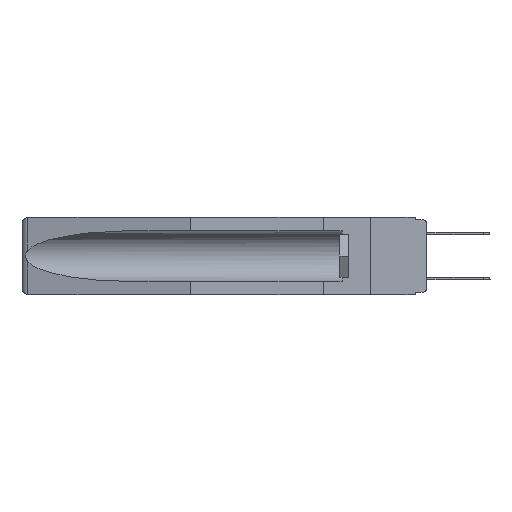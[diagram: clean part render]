
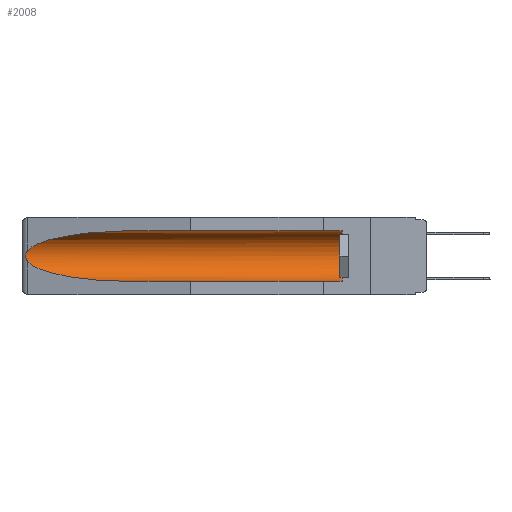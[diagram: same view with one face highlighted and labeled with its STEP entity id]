
A CAD part, left-side view. The second image highlights one B-rep face of the part: STEP entity #2008.
In plain terms, the highlighted cylindrical face has radius 2.857 mm (diameter 5.715 mm), a partial arc.
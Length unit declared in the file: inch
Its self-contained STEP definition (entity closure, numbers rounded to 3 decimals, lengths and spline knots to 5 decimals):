
#389 = ORIENTED_EDGE ( 'NONE', *, *, #9633, .T. ) ;
#558 = CARTESIAN_POINT ( 'NONE',  ( 0.26537, 1.52718, -0.14972 ) ) ;
#1494 = CARTESIAN_POINT ( 'NONE',  ( 0.21114, 1.30732, -0.284 ) ) ;
#1794 = CARTESIAN_POINT ( 'NONE',  ( 0.155, 0.126, -0.059 ) ) ;
#1816 = AXIS2_PLACEMENT_3D ( 'NONE', #8022, #11916, #23338 ) ;
#2008 = ADVANCED_FACE ( 'NONE', ( #5733 ), #3607, .F. ) ;
#2300 = EDGE_CURVE ( 'NONE', #23781, #16436, #9685, .T. ) ;
#2489 = CARTESIAN_POINT ( 'NONE',  ( 0.2675, 1.53308, -0.17534 ) ) ;
#2568 = CARTESIAN_POINT ( 'NONE',  ( 0.155, 1.07973, -0.284 ) ) ;
#2763 = CARTESIAN_POINT ( 'NONE',  ( 0.26597, 1.52961, -0.15275 ) ) ;
#3242 = DIRECTION ( 'NONE',  ( 0., 0., 1. ) ) ;
#3607 = CYLINDRICAL_SURFACE ( 'NONE', #19443, 0.1125 ) ;
#4563 = CARTESIAN_POINT ( 'NONE',  ( 0.155, -0.30754, -0.059 ) ) ;
#4999 = VERTEX_POINT ( 'NONE', #23494 ) ;
#5733 = FACE_OUTER_BOUND ( 'NONE', #6894, .T. ) ;
#6511 = CARTESIAN_POINT ( 'NONE',  ( 0.2675, 1.53308, -0.16763 ) ) ;
#6894 = EDGE_LOOP ( 'NONE', ( #14078, #10141, #15037, #9399, #17357, #389 ) ) ;
#6945 = CARTESIAN_POINT ( 'NONE',  ( 0.155, -0.30754, -0.284 ) ) ;
#7158 = LINE ( 'NONE', #4563, #17758 ) ;
#7520 =( BOUNDED_CURVE ( )  B_SPLINE_CURVE ( 3, ( #16853, #18918, #1494, #20624 ),
 .UNSPECIFIED., .F., .F. ) 
 B_SPLINE_CURVE_WITH_KNOTS ( ( 4, 4 ),
 ( 0.1948, 1.5708 ),
 .UNSPECIFIED. ) 
 CURVE ( )  GEOMETRIC_REPRESENTATION_ITEM ( )  RATIONAL_B_SPLINE_CURVE ( ( 1., 0.848, 0.848, 1. ) ) 
 REPRESENTATION_ITEM ( '' )  );
#8022 = CARTESIAN_POINT ( 'NONE',  ( 0.155, 0.126, -0.1715 ) ) ;
#8628 = CARTESIAN_POINT ( 'NONE',  ( 0.26654, 1.53092, -0.15636 ) ) ;
#9138 = CARTESIAN_POINT ( 'NONE',  ( 0.25451, 1.48313, -0.09465 ) ) ;
#9318 = VERTEX_POINT ( 'NONE', #1794 ) ;
#9399 = ORIENTED_EDGE ( 'NONE', *, *, #23241, .F. ) ;
#9633 = EDGE_CURVE ( 'NONE', #9318, #21368, #7158, .T. ) ;
#9685 = B_SPLINE_CURVE_WITH_KNOTS ( 'NONE', 3,
 ( #558, #2763, #8628, #14141, #6511, #2489, #18847, #22431, #16617, #14838 ),
 .UNSPECIFIED., .F., .F.,
 ( 4, 2, 2, 2, 4 ),
 ( 0., 0.00029, 0.00058, 0.00087, 0.00117 ),
 .UNSPECIFIED. ) ;
#9855 = VECTOR ( 'NONE', #12443, 39.37008 ) ;
#10141 = ORIENTED_EDGE ( 'NONE', *, *, #2300, .T. ) ;
#10389 = EDGE_CURVE ( 'NONE', #4999, #9318, #14377, .T. ) ;
#11916 = DIRECTION ( 'NONE',  ( 0., -1., 0. ) ) ;
#12443 = DIRECTION ( 'NONE',  ( 0., 1., 0. ) ) ;
#13778 = CARTESIAN_POINT ( 'NONE',  ( 0.26537, 1.52718, -0.19328 ) ) ;
#14078 = ORIENTED_EDGE ( 'NONE', *, *, #16100, .T. ) ;
#14141 = CARTESIAN_POINT ( 'NONE',  ( 0.2673, 1.5327, -0.16383 ) ) ;
#14180 = CARTESIAN_POINT ( 'NONE',  ( 0.26537, 1.52718, -0.14972 ) ) ;
#14377 = CIRCLE ( 'NONE', #1816, 0.1125 ) ;
#14838 = CARTESIAN_POINT ( 'NONE',  ( 0.26537, 1.52718, -0.19328 ) ) ;
#15034 = LINE ( 'NONE', #6945, #9855 ) ;
#15037 = ORIENTED_EDGE ( 'NONE', *, *, #16135, .T. ) ;
#16100 = EDGE_CURVE ( 'NONE', #21368, #23781, #24531, .T. ) ;
#16135 = EDGE_CURVE ( 'NONE', #16436, #21412, #7520, .T. ) ;
#16436 = VERTEX_POINT ( 'NONE', #13778 ) ;
#16455 = DIRECTION ( 'NONE',  ( 0., 1., 0. ) ) ;
#16617 = CARTESIAN_POINT ( 'NONE',  ( 0.26597, 1.5296, -0.19026 ) ) ;
#16772 = CARTESIAN_POINT ( 'NONE',  ( 0.21114, 1.30732, -0.059 ) ) ;
#16853 = CARTESIAN_POINT ( 'NONE',  ( 0.26537, 1.52718, -0.19328 ) ) ;
#17357 = ORIENTED_EDGE ( 'NONE', *, *, #10389, .T. ) ;
#17758 = VECTOR ( 'NONE', #16455, 39.37008 ) ;
#18654 = CARTESIAN_POINT ( 'NONE',  ( 0.155, 1.07973, -0.059 ) ) ;
#18847 = CARTESIAN_POINT ( 'NONE',  ( 0.2673, 1.53269, -0.17917 ) ) ;
#18918 = CARTESIAN_POINT ( 'NONE',  ( 0.25451, 1.48313, -0.24835 ) ) ;
#19443 = AXIS2_PLACEMENT_3D ( 'NONE', #22973, #24780, #3242 ) ;
#20624 = CARTESIAN_POINT ( 'NONE',  ( 0.155, 1.07973, -0.284 ) ) ;
#21368 = VERTEX_POINT ( 'NONE', #22163 ) ;
#21412 = VERTEX_POINT ( 'NONE', #2568 ) ;
#22163 = CARTESIAN_POINT ( 'NONE',  ( 0.155, 1.07973, -0.059 ) ) ;
#22431 = CARTESIAN_POINT ( 'NONE',  ( 0.26655, 1.53094, -0.18657 ) ) ;
#22750 = CARTESIAN_POINT ( 'NONE',  ( 0.26537, 1.52718, -0.14972 ) ) ;
#22973 = CARTESIAN_POINT ( 'NONE',  ( 0.155, -0.30754, -0.1715 ) ) ;
#23241 = EDGE_CURVE ( 'NONE', #4999, #21412, #15034, .T. ) ;
#23338 = DIRECTION ( 'NONE',  ( 0., 0., 1. ) ) ;
#23494 = CARTESIAN_POINT ( 'NONE',  ( 0.155, 0.126, -0.284 ) ) ;
#23781 = VERTEX_POINT ( 'NONE', #14180 ) ;
#24531 =( BOUNDED_CURVE ( )  B_SPLINE_CURVE ( 3, ( #18654, #16772, #9138, #22750 ),
 .UNSPECIFIED., .F., .F. ) 
 B_SPLINE_CURVE_WITH_KNOTS ( ( 4, 4 ),
 ( 4.71239, 6.08839 ),
 .UNSPECIFIED. ) 
 CURVE ( )  GEOMETRIC_REPRESENTATION_ITEM ( )  RATIONAL_B_SPLINE_CURVE ( ( 1., 0.848, 0.848, 1. ) ) 
 REPRESENTATION_ITEM ( '' )  );
#24780 = DIRECTION ( 'NONE',  ( 0., 1., 0. ) ) ;
